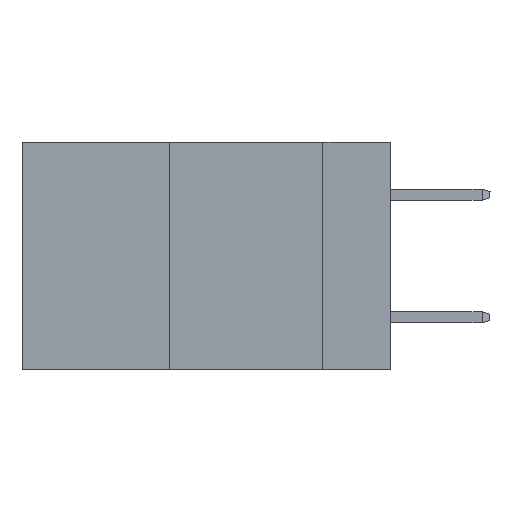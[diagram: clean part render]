
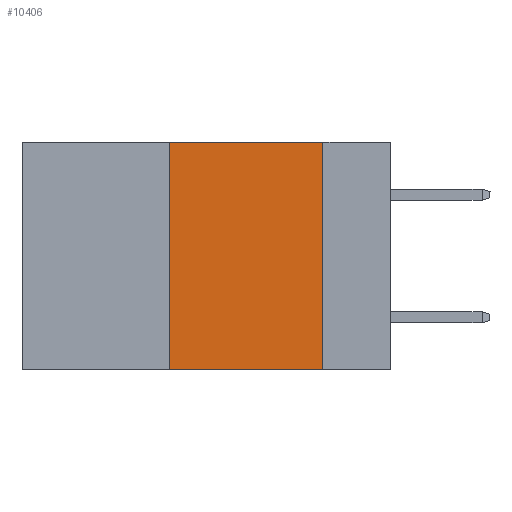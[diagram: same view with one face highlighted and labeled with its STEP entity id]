
A CAD part, left-side view. The second image highlights one B-rep face of the part: STEP entity #10406.
In plain terms, the highlighted planar face has unit normal (-1, 0, 0).
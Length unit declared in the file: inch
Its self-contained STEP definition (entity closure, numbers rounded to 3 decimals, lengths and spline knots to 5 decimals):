
#95 = EDGE_CURVE ( 'NONE', #10737, #18014, #16959, .T. ) ;
#559 = EDGE_CURVE ( 'NONE', #13572, #16467, #1673, .T. ) ;
#642 = DIRECTION ( 'NONE',  ( 0., 0., -1. ) ) ;
#1351 = CARTESIAN_POINT ( 'NONE',  ( 0., 0.11, -0.37 ) ) ;
#1673 = LINE ( 'NONE', #16066, #13182 ) ;
#2615 = DIRECTION ( 'NONE',  ( 0., -1., 0. ) ) ;
#3108 = DIRECTION ( 'NONE',  ( 0., 0., 1. ) ) ;
#3131 = EDGE_CURVE ( 'NONE', #10737, #13572, #4400, .T. ) ;
#3275 = CARTESIAN_POINT ( 'NONE',  ( 0., 0.36, 0. ) ) ;
#3850 = EDGE_CURVE ( 'NONE', #16467, #18014, #16630, .T. ) ;
#4183 = VECTOR ( 'NONE', #7002, 39.37008 ) ;
#4227 = CARTESIAN_POINT ( 'NONE',  ( 0., 0.6, -0.37 ) ) ;
#4400 = LINE ( 'NONE', #12024, #17092 ) ;
#4834 = ORIENTED_EDGE ( 'NONE', *, *, #95, .T. ) ;
#5356 = CARTESIAN_POINT ( 'NONE',  ( 0., 0.11, 0. ) ) ;
#5971 = ORIENTED_EDGE ( 'NONE', *, *, #559, .F. ) ;
#6464 = CARTESIAN_POINT ( 'NONE',  ( 0., 0.11, 0. ) ) ;
#7002 = DIRECTION ( 'NONE',  ( 0., 0., -1. ) ) ;
#7922 = PLANE ( 'NONE',  #18870 ) ;
#8022 = ORIENTED_EDGE ( 'NONE', *, *, #3131, .F. ) ;
#10406 = ADVANCED_FACE ( 'NONE', ( #12406 ), #7922, .F. ) ;
#10737 = VERTEX_POINT ( 'NONE', #11332 ) ;
#11332 = CARTESIAN_POINT ( 'NONE',  ( 0., 0.36, -0.37 ) ) ;
#12024 = CARTESIAN_POINT ( 'NONE',  ( 0., 0.36, 0. ) ) ;
#12406 = FACE_OUTER_BOUND ( 'NONE', #15744, .T. ) ;
#12581 = CARTESIAN_POINT ( 'NONE',  ( 0., 0.6, 0. ) ) ;
#13092 = ORIENTED_EDGE ( 'NONE', *, *, #3850, .F. ) ;
#13182 = VECTOR ( 'NONE', #2615, 39.37008 ) ;
#13572 = VERTEX_POINT ( 'NONE', #3275 ) ;
#15744 = EDGE_LOOP ( 'NONE', ( #13092, #5971, #8022, #4834 ) ) ;
#16066 = CARTESIAN_POINT ( 'NONE',  ( 0., 0.6, 0. ) ) ;
#16467 = VERTEX_POINT ( 'NONE', #6464 ) ;
#16630 = LINE ( 'NONE', #5356, #4183 ) ;
#16959 = LINE ( 'NONE', #4227, #17188 ) ;
#17092 = VECTOR ( 'NONE', #3108, 39.37008 ) ;
#17188 = VECTOR ( 'NONE', #19190, 39.37008 ) ;
#18014 = VERTEX_POINT ( 'NONE', #1351 ) ;
#18527 = DIRECTION ( 'NONE',  ( 1., 0., 0. ) ) ;
#18870 = AXIS2_PLACEMENT_3D ( 'NONE', #12581, #18527, #642 ) ;
#19190 = DIRECTION ( 'NONE',  ( 0., -1., 0. ) ) ;
